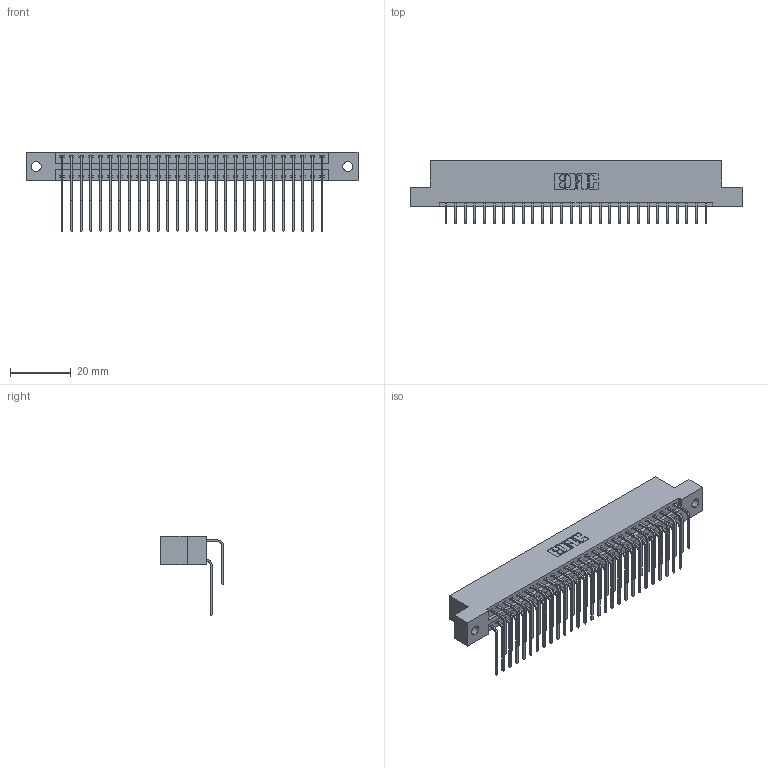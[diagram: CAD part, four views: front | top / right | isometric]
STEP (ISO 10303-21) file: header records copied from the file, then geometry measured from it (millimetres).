
FILE_DESCRIPTION (( 'STEP AP203' ), '1' );
FILE_NAME ('396-056-559-202.STEP', '2019-11-03T09:19:59', ( '' ), ( '' ), 'SwSTEP 2.0', 'SolidWorks 2016', '' );
FILE_SCHEMA (( 'CONFIG_CONTROL_DESIGN' ));
Length unit declared in the file: inch
Products named in the file (4): 346 Part_Flush Mounting Lugs - 0.128 Dia; 345-292-001_559 Tail - 2; 396-056-559-202; 345-292-001_558 559 Tail - 1
Assembly tree (57 placements, depth 2):
  396-056-559-202
    346 Part_Flush Mounting Lugs - 0.128 Dia
    345-292-001_558 559 Tail - 1  x28
    345-292-001_559 Tail - 2  x28
Bounding box: 109.47 x 20.89 x 26.16 mm (x, y, z)
Volume: 10852.7 mm3; surface area: 15978.3 mm2
Topology: 57 solids, 57 shells, 3146 faces, 9345 edges, 6154 vertices
Faces by surface type: plane 2148, cylinder 998
Entity records: 21945 total; most frequent: CARTESIAN_POINT 3687, ORIENTED_EDGE 3570, DIRECTION 3273, EDGE_CURVE 1785, LINE 1501, VECTOR 1501, VERTEX_POINT 1186, AXIS2_PLACEMENT_3D 886
